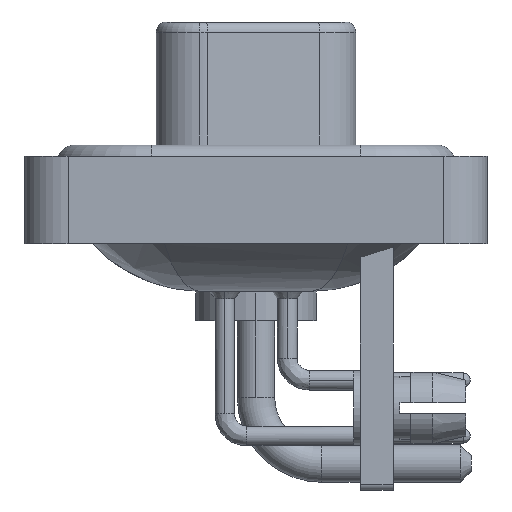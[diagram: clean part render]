
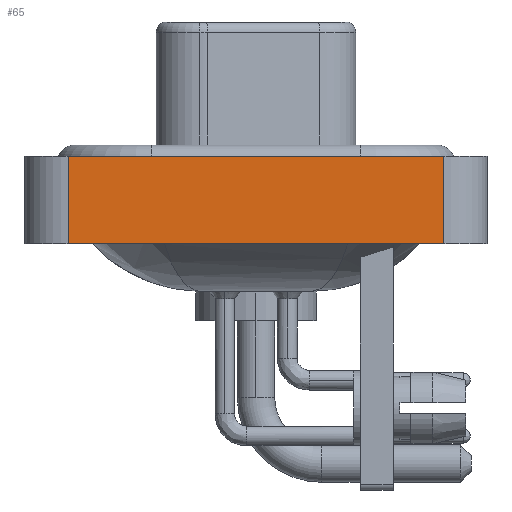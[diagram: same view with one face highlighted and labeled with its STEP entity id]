
A CAD part, left-side view. The second image highlights one B-rep face of the part: STEP entity #65.
In plain terms, the highlighted planar face has unit normal (-1, 0, 0).
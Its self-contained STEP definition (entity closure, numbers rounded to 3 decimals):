
#1 = CARTESIAN_POINT ( 'NONE',  ( -7.25, 8.55, -3.6 ) ) ;
#65 = ADVANCED_FACE ( 'NONE', ( #11143 ), #16863, .T. ) ;
#460 = CARTESIAN_POINT ( 'NONE',  ( -7.25, -8.55, -3.6 ) ) ;
#493 = DIRECTION ( 'NONE',  ( 0., -1., 0. ) ) ;
#591 = LINE ( 'NONE', #8232, #9424 ) ;
#1754 = CARTESIAN_POINT ( 'NONE',  ( -7.25, -8.55, -3.6 ) ) ;
#2573 = LINE ( 'NONE', #8533, #3018 ) ;
#2612 = LINE ( 'NONE', #460, #15952 ) ;
#3018 = VECTOR ( 'NONE', #10323, 1000. ) ;
#3513 = CARTESIAN_POINT ( 'NONE',  ( -7.25, -8.55, 0.4 ) ) ;
#4398 = VERTEX_POINT ( 'NONE', #3513 ) ;
#5146 = EDGE_CURVE ( 'NONE', #21944, #4398, #2573, .T. ) ;
#6075 = LINE ( 'NONE', #11677, #23085 ) ;
#8232 = CARTESIAN_POINT ( 'NONE',  ( -7.25, 8.55, -3.6 ) ) ;
#8533 = CARTESIAN_POINT ( 'NONE',  ( -7.25, -8.55, -3.6 ) ) ;
#9424 = VECTOR ( 'NONE', #9743, 1000. ) ;
#9743 = DIRECTION ( 'NONE',  ( 0., 0., 1. ) ) ;
#10189 = VERTEX_POINT ( 'NONE', #23826 ) ;
#10323 = DIRECTION ( 'NONE',  ( 0., 0., 1. ) ) ;
#10644 = VERTEX_POINT ( 'NONE', #1 ) ;
#10734 = DIRECTION ( 'NONE',  ( 0., 0., 1. ) ) ;
#10892 = ORIENTED_EDGE ( 'NONE', *, *, #12411, .T. ) ;
#11143 = FACE_OUTER_BOUND ( 'NONE', #18878, .T. ) ;
#11677 = CARTESIAN_POINT ( 'NONE',  ( -7.25, -8.55, 0.4 ) ) ;
#12411 = EDGE_CURVE ( 'NONE', #10644, #21944, #2612, .T. ) ;
#12899 = DIRECTION ( 'NONE',  ( -1., 0., 0. ) ) ;
#13240 = ORIENTED_EDGE ( 'NONE', *, *, #5146, .T. ) ;
#13512 = ORIENTED_EDGE ( 'NONE', *, *, #14793, .F. ) ;
#14793 = EDGE_CURVE ( 'NONE', #10189, #4398, #6075, .T. ) ;
#15952 = VECTOR ( 'NONE', #22397, 1000. ) ;
#16863 = PLANE ( 'NONE',  #19475 ) ;
#17921 = EDGE_CURVE ( 'NONE', #10644, #10189, #591, .T. ) ;
#18280 = CARTESIAN_POINT ( 'NONE',  ( -7.25, -8.55, -3.6 ) ) ;
#18760 = ORIENTED_EDGE ( 'NONE', *, *, #17921, .F. ) ;
#18878 = EDGE_LOOP ( 'NONE', ( #13240, #13512, #18760, #10892 ) ) ;
#19475 = AXIS2_PLACEMENT_3D ( 'NONE', #18280, #12899, #10734 ) ;
#21944 = VERTEX_POINT ( 'NONE', #1754 ) ;
#22397 = DIRECTION ( 'NONE',  ( 0., -1., 0. ) ) ;
#23085 = VECTOR ( 'NONE', #493, 1000. ) ;
#23826 = CARTESIAN_POINT ( 'NONE',  ( -7.25, 8.55, 0.4 ) ) ;
